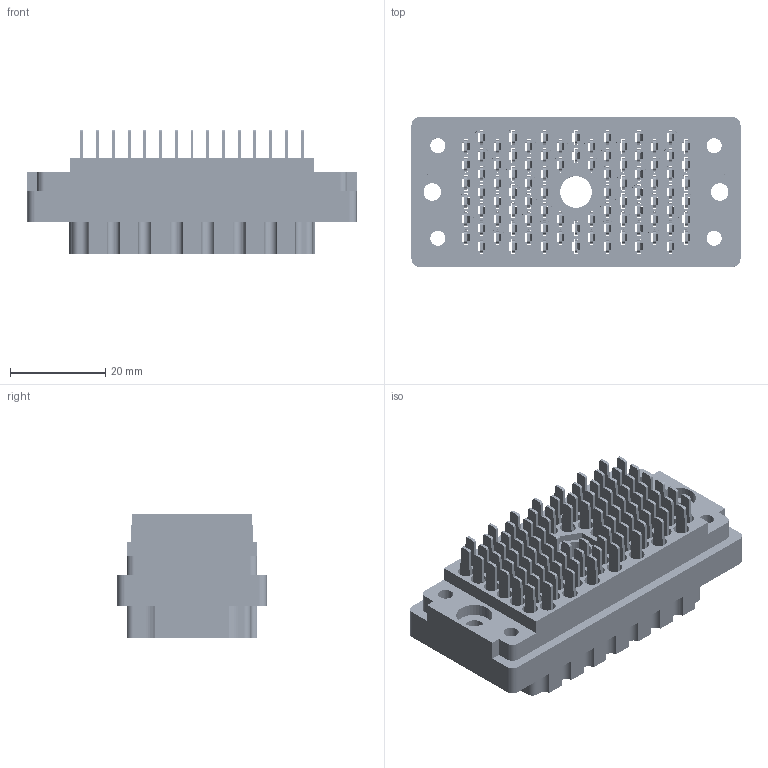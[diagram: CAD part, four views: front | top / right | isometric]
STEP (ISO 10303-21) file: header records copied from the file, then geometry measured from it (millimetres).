
FILE_DESCRIPTION (( 'STEP AP203' ), '1' );
FILE_NAME ('516-090-501-400.STEP', '2020-09-08T17:56:44', ( '' ), ( '' ), 'SwSTEP 2.0', 'SolidWorks 2020', '' );
FILE_SCHEMA (( 'CONFIG_CONTROL_DESIGN' ));
Length unit declared in the file: inch
Products named in the file (3): 516 Part Receptacle_090; 516-292-001_501 Contact; 516-090-501-400
Assembly tree (92 placements, depth 2):
  516-090-501-400
    516 Part Receptacle_090
    516-292-001_501 Contact  x91
Bounding box: 69.04 x 31.34 x 26.21 mm (x, y, z)
Volume: 23465.1 mm3; surface area: 46321.4 mm2
Topology: 92 solids, 92 shells, 8476 faces, 24642 edges, 16366 vertices
Faces by surface type: plane 5106, cylinder 2822, bspline 546, cone 2
Entity records: 70628 total; most frequent: CARTESIAN_POINT 12244, ORIENTED_EDGE 11844, DIRECTION 11554, EDGE_CURVE 5922, VECTOR 4392, LINE 4392, VERTEX_POINT 3946, AXIS2_PLACEMENT_3D 3581
